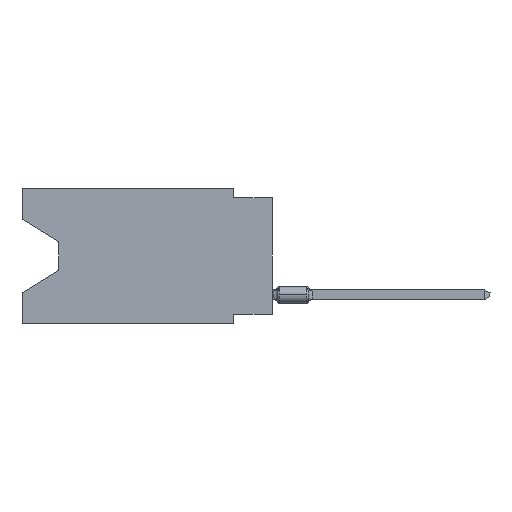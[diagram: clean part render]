
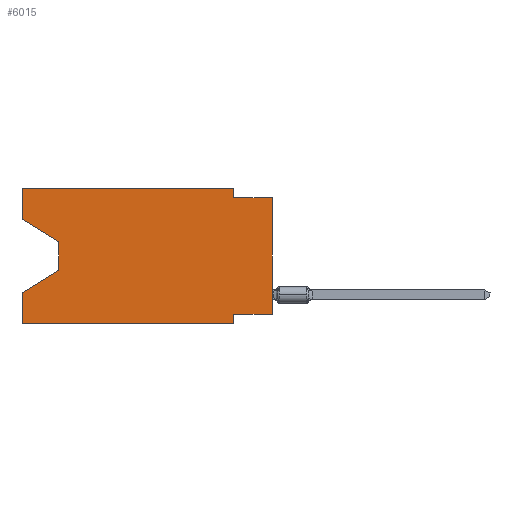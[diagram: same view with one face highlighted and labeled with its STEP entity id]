
A CAD part, left-side view. The second image highlights one B-rep face of the part: STEP entity #6015.
In plain terms, the highlighted planar face has unit normal (-1, 0, 0).
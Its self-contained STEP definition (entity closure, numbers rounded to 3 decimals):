
#926 = VERTEX_POINT ( 'NONE', #13611 ) ;
#1324 = EDGE_CURVE ( 'NONE', #10877, #28471, #29153, .T. ) ;
#1444 = ORIENTED_EDGE ( 'NONE', *, *, #31703, .F. ) ;
#1574 = EDGE_CURVE ( 'NONE', #36311, #16034, #38077, .T. ) ;
#1802 = CARTESIAN_POINT ( 'NONE',  ( 0., 16.383, 0. ) ) ;
#1898 = VECTOR ( 'NONE', #26882, 1000. ) ;
#1904 = CARTESIAN_POINT ( 'NONE',  ( 0., 2.54, -8.89 ) ) ;
#2243 = LINE ( 'NONE', #5411, #32671 ) ;
#3112 = VERTEX_POINT ( 'NONE', #19545 ) ;
#3451 = ORIENTED_EDGE ( 'NONE', *, *, #12842, .F. ) ;
#3889 = ORIENTED_EDGE ( 'NONE', *, *, #25490, .T. ) ;
#4444 = VERTEX_POINT ( 'NONE', #26560 ) ;
#5087 = VECTOR ( 'NONE', #5730, 1000. ) ;
#5411 = CARTESIAN_POINT ( 'NONE',  ( 0., 16.383, -2.038 ) ) ;
#5473 = VECTOR ( 'NONE', #31996, 1000. ) ;
#5644 = LINE ( 'NONE', #38262, #34233 ) ;
#5719 = LINE ( 'NONE', #20380, #33427 ) ;
#5730 = DIRECTION ( 'NONE',  ( 0., 0., -1. ) ) ;
#6015 = ADVANCED_FACE ( 'NONE', ( #25940 ), #31472, .F. ) ;
#6198 = CARTESIAN_POINT ( 'NONE',  ( 0., 2.54, -8.255 ) ) ;
#7622 = DIRECTION ( 'NONE',  ( 0., 0., -1. ) ) ;
#8134 = DIRECTION ( 'NONE',  ( 0., 0., -1. ) ) ;
#9448 = CARTESIAN_POINT ( 'NONE',  ( 0., 13.97, -5.385 ) ) ;
#9829 = VECTOR ( 'NONE', #38252, 1000. ) ;
#10877 = VERTEX_POINT ( 'NONE', #22535 ) ;
#10959 = ORIENTED_EDGE ( 'NONE', *, *, #22279, .F. ) ;
#11587 = DIRECTION ( 'NONE',  ( 0., -1., 0. ) ) ;
#12842 = EDGE_CURVE ( 'NONE', #926, #3112, #5719, .T. ) ;
#13274 = CARTESIAN_POINT ( 'NONE',  ( 0., 2.54, -0.635 ) ) ;
#13611 = CARTESIAN_POINT ( 'NONE',  ( 0., 16.383, 0. ) ) ;
#13629 = VECTOR ( 'NONE', #7622, 1000. ) ;
#14315 = DIRECTION ( 'NONE',  ( 0., -0.855, -0.519 ) ) ;
#14526 = CARTESIAN_POINT ( 'NONE',  ( 0., 13.97, -5.385 ) ) ;
#15549 = VECTOR ( 'NONE', #26830, 1000. ) ;
#16034 = VERTEX_POINT ( 'NONE', #36993 ) ;
#16199 = VECTOR ( 'NONE', #32539, 1000. ) ;
#16791 = LINE ( 'NONE', #17559, #5473 ) ;
#17043 = ORIENTED_EDGE ( 'NONE', *, *, #32331, .T. ) ;
#17220 = CARTESIAN_POINT ( 'NONE',  ( 0., 16.383, 0. ) ) ;
#17559 = CARTESIAN_POINT ( 'NONE',  ( 0., 0., -0.635 ) ) ;
#17630 = VERTEX_POINT ( 'NONE', #29857 ) ;
#17747 = VERTEX_POINT ( 'NONE', #13274 ) ;
#18332 = LINE ( 'NONE', #36305, #15549 ) ;
#18339 = EDGE_LOOP ( 'NONE', ( #3889, #36105, #17043, #29229, #32246, #26414, #10959, #31367, #24376, #1444, #3451, #37619 ) ) ;
#18682 = AXIS2_PLACEMENT_3D ( 'NONE', #1802, #38168, #8134 ) ;
#19545 = CARTESIAN_POINT ( 'NONE',  ( 0., 2.54, 0. ) ) ;
#19887 = LINE ( 'NONE', #22864, #36293 ) ;
#20084 = LINE ( 'NONE', #32524, #9829 ) ;
#20380 = CARTESIAN_POINT ( 'NONE',  ( 0., 16.383, 0. ) ) ;
#20508 = EDGE_CURVE ( 'NONE', #17747, #4444, #16791, .T. ) ;
#22067 = EDGE_CURVE ( 'NONE', #25289, #4444, #18332, .T. ) ;
#22279 = EDGE_CURVE ( 'NONE', #25289, #36311, #20084, .T. ) ;
#22329 = EDGE_CURVE ( 'NONE', #33286, #29245, #19887, .T. ) ;
#22535 = CARTESIAN_POINT ( 'NONE',  ( 0., 13.97, -3.505 ) ) ;
#22864 = CARTESIAN_POINT ( 'NONE',  ( 0., 16.383, 0. ) ) ;
#23491 = CARTESIAN_POINT ( 'NONE',  ( 0., 16.383, -6.852 ) ) ;
#24376 = ORIENTED_EDGE ( 'NONE', *, *, #20508, .F. ) ;
#24890 = DIRECTION ( 'NONE',  ( 0., 0.855, -0.519 ) ) ;
#25289 = VERTEX_POINT ( 'NONE', #34884 ) ;
#25490 = EDGE_CURVE ( 'NONE', #17630, #10877, #2243, .T. ) ;
#25818 = CARTESIAN_POINT ( 'NONE',  ( 0., 13.97, -3.505 ) ) ;
#25940 = FACE_OUTER_BOUND ( 'NONE', #18339, .T. ) ;
#26022 = DIRECTION ( 'NONE',  ( 0., 0., 1. ) ) ;
#26414 = ORIENTED_EDGE ( 'NONE', *, *, #1574, .F. ) ;
#26560 = CARTESIAN_POINT ( 'NONE',  ( 0., 0., -0.635 ) ) ;
#26830 = DIRECTION ( 'NONE',  ( 0., 0., 1. ) ) ;
#26882 = DIRECTION ( 'NONE',  ( 0., 0., 1. ) ) ;
#27833 = LINE ( 'NONE', #9448, #38576 ) ;
#28471 = VERTEX_POINT ( 'NONE', #14526 ) ;
#29153 = LINE ( 'NONE', #25818, #13629 ) ;
#29229 = ORIENTED_EDGE ( 'NONE', *, *, #22329, .F. ) ;
#29245 = VERTEX_POINT ( 'NONE', #23491 ) ;
#29460 = LINE ( 'NONE', #17220, #1898 ) ;
#29857 = CARTESIAN_POINT ( 'NONE',  ( 0., 16.383, -2.038 ) ) ;
#30488 = EDGE_CURVE ( 'NONE', #17630, #926, #29460, .T. ) ;
#31367 = ORIENTED_EDGE ( 'NONE', *, *, #22067, .T. ) ;
#31472 = PLANE ( 'NONE',  #18682 ) ;
#31703 = EDGE_CURVE ( 'NONE', #3112, #17747, #32812, .T. ) ;
#31996 = DIRECTION ( 'NONE',  ( 0., -1., 0. ) ) ;
#32246 = ORIENTED_EDGE ( 'NONE', *, *, #32657, .T. ) ;
#32331 = EDGE_CURVE ( 'NONE', #28471, #29245, #27833, .T. ) ;
#32524 = CARTESIAN_POINT ( 'NONE',  ( 0., 0., -8.255 ) ) ;
#32539 = DIRECTION ( 'NONE',  ( 0., 0., -1. ) ) ;
#32657 = EDGE_CURVE ( 'NONE', #33286, #16034, #5644, .T. ) ;
#32671 = VECTOR ( 'NONE', #14315, 1000. ) ;
#32812 = LINE ( 'NONE', #35392, #5087 ) ;
#33286 = VERTEX_POINT ( 'NONE', #37029 ) ;
#33427 = VECTOR ( 'NONE', #36156, 1000. ) ;
#34233 = VECTOR ( 'NONE', #11587, 1000. ) ;
#34884 = CARTESIAN_POINT ( 'NONE',  ( 0., 0., -8.255 ) ) ;
#35392 = CARTESIAN_POINT ( 'NONE',  ( 0., 2.54, 0. ) ) ;
#36105 = ORIENTED_EDGE ( 'NONE', *, *, #1324, .T. ) ;
#36156 = DIRECTION ( 'NONE',  ( 0., -1., 0. ) ) ;
#36293 = VECTOR ( 'NONE', #26022, 1000. ) ;
#36305 = CARTESIAN_POINT ( 'NONE',  ( 0., 0., 0. ) ) ;
#36311 = VERTEX_POINT ( 'NONE', #6198 ) ;
#36993 = CARTESIAN_POINT ( 'NONE',  ( 0., 2.54, -8.89 ) ) ;
#37029 = CARTESIAN_POINT ( 'NONE',  ( 0., 16.383, -8.89 ) ) ;
#37619 = ORIENTED_EDGE ( 'NONE', *, *, #30488, .F. ) ;
#38077 = LINE ( 'NONE', #1904, #16199 ) ;
#38168 = DIRECTION ( 'NONE',  ( 1., 0., 0. ) ) ;
#38252 = DIRECTION ( 'NONE',  ( 0., 1., 0. ) ) ;
#38262 = CARTESIAN_POINT ( 'NONE',  ( 0., 16.383, -8.89 ) ) ;
#38576 = VECTOR ( 'NONE', #24890, 1000. ) ;
